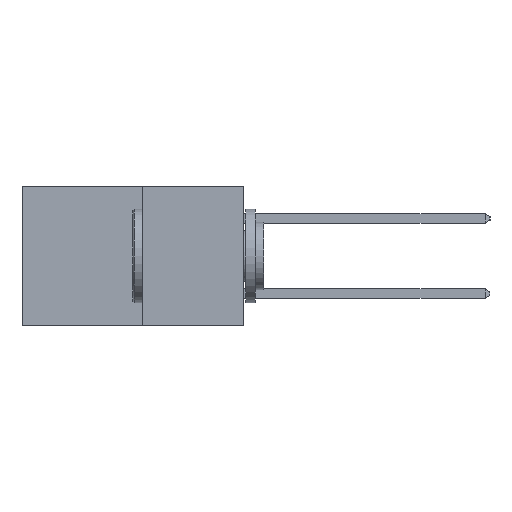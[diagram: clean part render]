
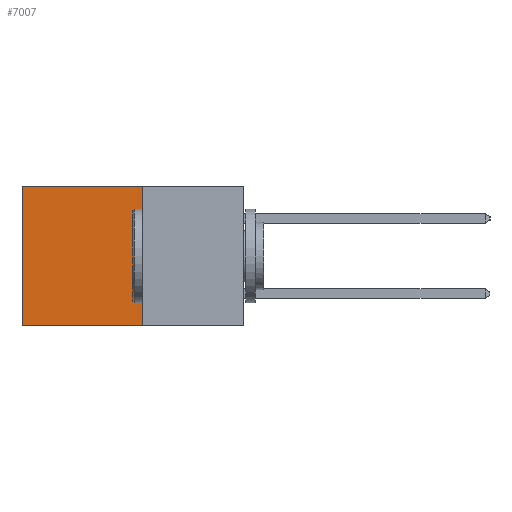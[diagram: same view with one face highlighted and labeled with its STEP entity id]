
A CAD part, left-side view. The second image highlights one B-rep face of the part: STEP entity #7007.
In plain terms, the highlighted planar face has unit normal (-1, 0, 0).
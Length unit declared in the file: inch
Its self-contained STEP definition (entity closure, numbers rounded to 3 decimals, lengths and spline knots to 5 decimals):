
#503 = VECTOR ( 'NONE', #4981, 39.37008 ) ;
#660 = VERTEX_POINT ( 'NONE', #845 ) ;
#787 = LINE ( 'NONE', #5988, #503 ) ;
#798 = LINE ( 'NONE', #2480, #10165 ) ;
#845 = CARTESIAN_POINT ( 'NONE',  ( 0.277, 0.27, -0.37 ) ) ;
#1985 = VERTEX_POINT ( 'NONE', #7347 ) ;
#2218 = CARTESIAN_POINT ( 'NONE',  ( 0.277, 0.27, 0. ) ) ;
#2436 = AXIS2_PLACEMENT_3D ( 'NONE', #11287, #11075, #11014 ) ;
#2447 = VECTOR ( 'NONE', #6865, 39.37008 ) ;
#2480 = CARTESIAN_POINT ( 'NONE',  ( 0.277, 0.59, -0.37 ) ) ;
#2856 = ORIENTED_EDGE ( 'NONE', *, *, #10805, .F. ) ;
#3383 = EDGE_LOOP ( 'NONE', ( #5293, #7716, #2856, #11630 ) ) ;
#3500 = VERTEX_POINT ( 'NONE', #10470 ) ;
#4013 = VECTOR ( 'NONE', #6489, 39.37008 ) ;
#4027 = LINE ( 'NONE', #5949, #2447 ) ;
#4744 = DIRECTION ( 'NONE',  ( 0., 0., -1. ) ) ;
#4981 = DIRECTION ( 'NONE',  ( 0., 1., 0. ) ) ;
#5293 = ORIENTED_EDGE ( 'NONE', *, *, #6347, .T. ) ;
#5583 = CARTESIAN_POINT ( 'NONE',  ( 0.277, 0.27, 0. ) ) ;
#5783 = FACE_OUTER_BOUND ( 'NONE', #3383, .T. ) ;
#5949 = CARTESIAN_POINT ( 'NONE',  ( 0.277, 0.27, -0.37 ) ) ;
#5988 = CARTESIAN_POINT ( 'NONE',  ( 0.277, 0.27, -0.37 ) ) ;
#6145 = LINE ( 'NONE', #5583, #4013 ) ;
#6347 = EDGE_CURVE ( 'NONE', #3500, #1985, #798, .T. ) ;
#6489 = DIRECTION ( 'NONE',  ( 0., 1., 0. ) ) ;
#6784 = EDGE_CURVE ( 'NONE', #660, #1985, #787, .T. ) ;
#6865 = DIRECTION ( 'NONE',  ( 0., 0., -1. ) ) ;
#7007 = ADVANCED_FACE ( 'NONE', ( #5783 ), #10949, .F. ) ;
#7301 = VERTEX_POINT ( 'NONE', #2218 ) ;
#7347 = CARTESIAN_POINT ( 'NONE',  ( 0.277, 0.59, -0.37 ) ) ;
#7716 = ORIENTED_EDGE ( 'NONE', *, *, #6784, .F. ) ;
#10165 = VECTOR ( 'NONE', #4744, 39.37008 ) ;
#10470 = CARTESIAN_POINT ( 'NONE',  ( 0.277, 0.59, 0. ) ) ;
#10805 = EDGE_CURVE ( 'NONE', #7301, #660, #4027, .T. ) ;
#10949 = PLANE ( 'NONE',  #2436 ) ;
#11014 = DIRECTION ( 'NONE',  ( 0., 0., -1. ) ) ;
#11075 = DIRECTION ( 'NONE',  ( 1., 0., 0. ) ) ;
#11287 = CARTESIAN_POINT ( 'NONE',  ( 0.277, 0.27, -0.37 ) ) ;
#11484 = EDGE_CURVE ( 'NONE', #7301, #3500, #6145, .T. ) ;
#11630 = ORIENTED_EDGE ( 'NONE', *, *, #11484, .T. ) ;
